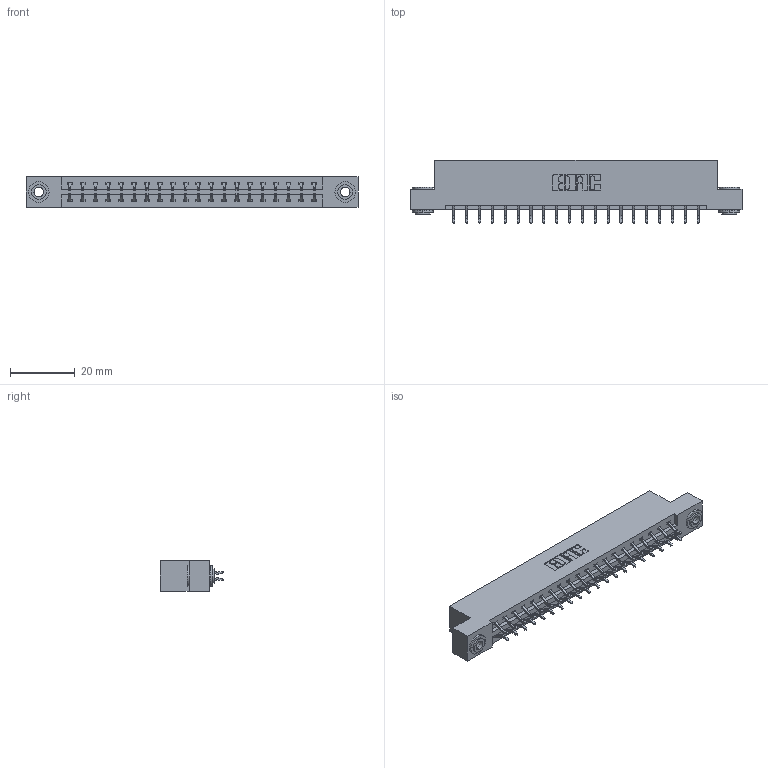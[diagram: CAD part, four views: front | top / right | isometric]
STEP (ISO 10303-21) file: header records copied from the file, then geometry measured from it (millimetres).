
FILE_DESCRIPTION (( 'STEP AP203' ), '1' );
FILE_NAME ('387-040-556-203.STEP', '2018-09-19T16:56:17', ( '' ), ( '' ), 'SwSTEP 2.0', 'SolidWorks 2016', '' );
FILE_SCHEMA (( 'CONFIG_CONTROL_DESIGN' ));
Length unit declared in the file: inch
Products named in the file (4): 345-250-002_345-250-002-102; 387-040-556-203; 337 Part_Flush Mounting Lugs - 0.156 Dia-TH; 345-292-001_556 Tail
Assembly tree (43 placements, depth 2):
  387-040-556-203
    337 Part_Flush Mounting Lugs - 0.156 Dia-TH
    345-292-001_556 Tail  x40
    345-250-002_345-250-002-102  x2
Bounding box: 102.26 x 19.57 x 9.4 mm (x, y, z)
Volume: 10502 mm3; surface area: 11841 mm2
Topology: 43 solids, 43 shells, 2552 faces, 7547 edges, 4974 vertices
Faces by surface type: plane 1760, cylinder 784, cone 8
Entity records: 19222 total; most frequent: CARTESIAN_POINT 3245, ORIENTED_EDGE 3162, DIRECTION 2823, EDGE_CURVE 1581, LINE 1421, VECTOR 1421, VERTEX_POINT 1050, AXIS2_PLACEMENT_3D 701
